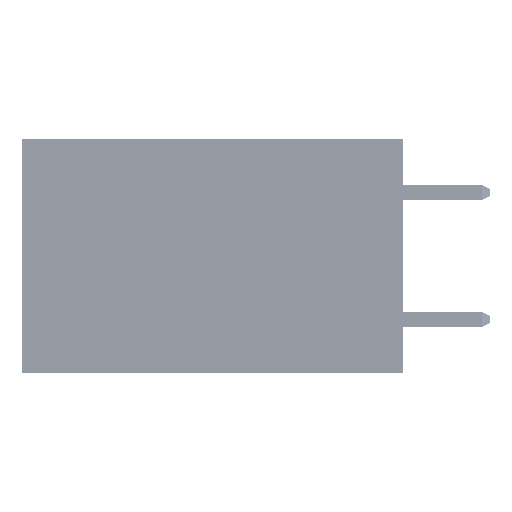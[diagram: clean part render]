
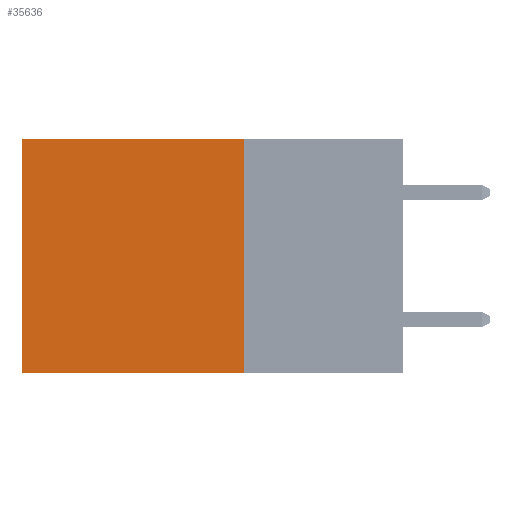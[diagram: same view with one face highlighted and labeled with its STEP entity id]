
A CAD part, left-side view. The second image highlights one B-rep face of the part: STEP entity #35636.
In plain terms, the highlighted planar face has unit normal (-1, 0, 0).
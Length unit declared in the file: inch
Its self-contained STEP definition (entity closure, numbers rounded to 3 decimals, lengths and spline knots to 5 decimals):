
#2374 = ORIENTED_EDGE ( 'NONE', *, *, #31515, .T. ) ;
#2943 = CARTESIAN_POINT ( 'NONE',  ( 0.2875, 0.6, 0. ) ) ;
#3542 = CARTESIAN_POINT ( 'NONE',  ( 0.2875, 0.25, -0.37 ) ) ;
#4178 = EDGE_CURVE ( 'NONE', #23264, #8810, #31054, .T. ) ;
#4298 = CARTESIAN_POINT ( 'NONE',  ( 0.2875, 0.25, 0. ) ) ;
#6105 = VECTOR ( 'NONE', #40539, 39.37008 ) ;
#8609 = CARTESIAN_POINT ( 'NONE',  ( 0.2875, 0.25, 0. ) ) ;
#8810 = VERTEX_POINT ( 'NONE', #12673 ) ;
#9508 = DIRECTION ( 'NONE',  ( 0., 1., 0. ) ) ;
#10725 = CARTESIAN_POINT ( 'NONE',  ( 0.2875, 0.25, -0.37 ) ) ;
#11050 = VECTOR ( 'NONE', #36975, 39.37008 ) ;
#12426 = DIRECTION ( 'NONE',  ( 1., 0., 0. ) ) ;
#12510 = VECTOR ( 'NONE', #9508, 39.37008 ) ;
#12673 = CARTESIAN_POINT ( 'NONE',  ( 0.2875, 0.6, -0.37 ) ) ;
#13313 = VERTEX_POINT ( 'NONE', #26194 ) ;
#13359 = CARTESIAN_POINT ( 'NONE',  ( 0.2875, 0.6, 0. ) ) ;
#16144 = LINE ( 'NONE', #2943, #6105 ) ;
#16540 = LINE ( 'NONE', #4298, #25363 ) ;
#23264 = VERTEX_POINT ( 'NONE', #3542 ) ;
#23573 = ORIENTED_EDGE ( 'NONE', *, *, #33153, .T. ) ;
#25363 = VECTOR ( 'NONE', #34321, 39.37008 ) ;
#26194 = CARTESIAN_POINT ( 'NONE',  ( 0.2875, 0.25, 0. ) ) ;
#27490 = ORIENTED_EDGE ( 'NONE', *, *, #4178, .F. ) ;
#29666 = FACE_OUTER_BOUND ( 'NONE', #43992, .T. ) ;
#29811 = EDGE_CURVE ( 'NONE', #13313, #23264, #16540, .T. ) ;
#31054 = LINE ( 'NONE', #10725, #11050 ) ;
#31124 = PLANE ( 'NONE',  #41613 ) ;
#31515 = EDGE_CURVE ( 'NONE', #44209, #8810, #16144, .T. ) ;
#32448 = LINE ( 'NONE', #46903, #12510 ) ;
#33153 = EDGE_CURVE ( 'NONE', #13313, #44209, #32448, .T. ) ;
#34321 = DIRECTION ( 'NONE',  ( 0., 0., -1. ) ) ;
#35636 = ADVANCED_FACE ( 'NONE', ( #29666 ), #31124, .F. ) ;
#36975 = DIRECTION ( 'NONE',  ( 0., 1., 0. ) ) ;
#38651 = DIRECTION ( 'NONE',  ( 0., 0., -1. ) ) ;
#40539 = DIRECTION ( 'NONE',  ( 0., 0., -1. ) ) ;
#41613 = AXIS2_PLACEMENT_3D ( 'NONE', #8609, #12426, #38651 ) ;
#43992 = EDGE_LOOP ( 'NONE', ( #2374, #27490, #46038, #23573 ) ) ;
#44209 = VERTEX_POINT ( 'NONE', #13359 ) ;
#46038 = ORIENTED_EDGE ( 'NONE', *, *, #29811, .F. ) ;
#46903 = CARTESIAN_POINT ( 'NONE',  ( 0.2875, 0.25, 0. ) ) ;
